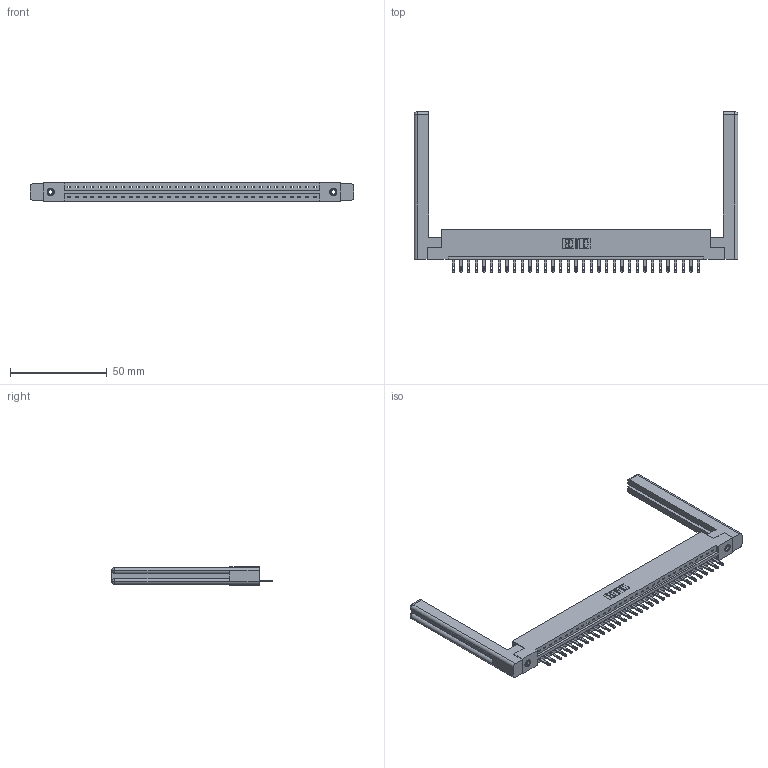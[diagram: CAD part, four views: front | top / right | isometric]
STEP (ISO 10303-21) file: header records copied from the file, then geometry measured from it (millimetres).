
FILE_DESCRIPTION (( 'STEP AP203' ), '1' );
FILE_NAME ('337-033-500-158.STEP', '2019-10-01T03:58:23', ( '' ), ( '' ), 'SwSTEP 2.0', 'SolidWorks 2016', '' );
FILE_SCHEMA (( 'CONFIG_CONTROL_DESIGN' ));
Length unit declared in the file: inch
Products named in the file (5): 337 Part_Flush Mounting Lugs - 0.156 Dia-TI; 345-250-001_345-250-001-102; 307-220-058; 337-033-500-158; 345-292-001_345-293-100
Assembly tree (38 placements, depth 2):
  337-033-500-158
    337 Part_Flush Mounting Lugs - 0.156 Dia-TI
    345-292-001_345-293-100  x33
    345-250-001_345-250-001-102  x2
    307-220-058  x2
Bounding box: 167.39 x 82.94 x 9.4 mm (x, y, z)
Volume: 24466.9 mm3; surface area: 23122 mm2
Topology: 38 solids, 38 shells, 2170 faces, 6605 edges, 4390 vertices
Faces by surface type: plane 1474, cylinder 672, cone 12, torus 12
Entity records: 28258 total; most frequent: CARTESIAN_POINT 4920, ORIENTED_EDGE 4828, DIRECTION 4180, EDGE_CURVE 2414, LINE 2234, VECTOR 2234, VERTEX_POINT 1602, AXIS2_PLACEMENT_3D 973
